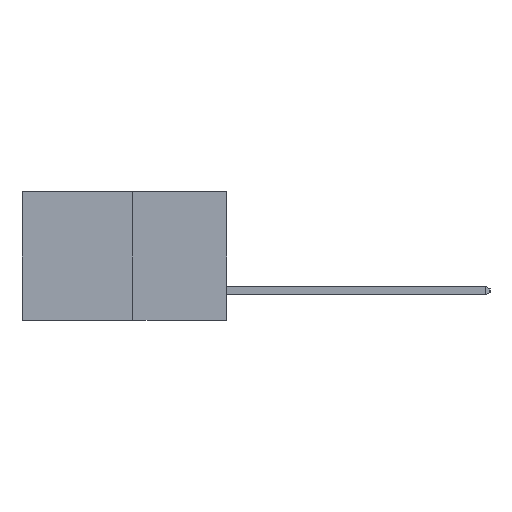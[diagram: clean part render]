
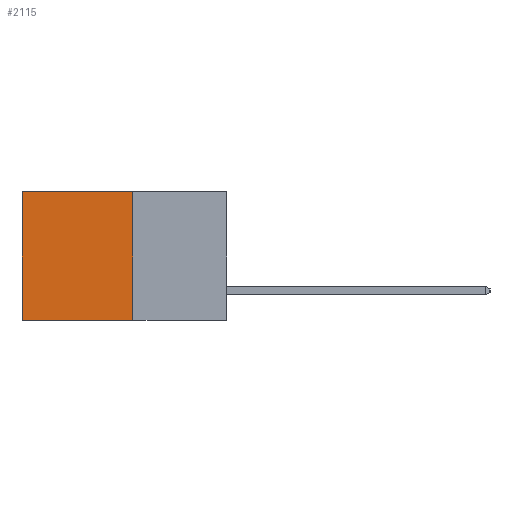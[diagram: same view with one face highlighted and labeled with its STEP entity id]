
A CAD part, left-side view. The second image highlights one B-rep face of the part: STEP entity #2115.
In plain terms, the highlighted planar face has unit normal (-1, 0, 0).
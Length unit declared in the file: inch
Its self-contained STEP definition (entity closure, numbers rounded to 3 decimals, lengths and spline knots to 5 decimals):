
#519 = ORIENTED_EDGE ( 'NONE', *, *, #10132, .F. ) ;
#786 = ORIENTED_EDGE ( 'NONE', *, *, #15309, .T. ) ;
#1230 = CARTESIAN_POINT ( 'NONE',  ( 0.277, 0.27, -0.37 ) ) ;
#1378 = ORIENTED_EDGE ( 'NONE', *, *, #7755, .F. ) ;
#1623 = EDGE_CURVE ( 'NONE', #3369, #8069, #8534, .T. ) ;
#2115 = ADVANCED_FACE ( 'NONE', ( #7200 ), #9930, .F. ) ;
#3288 = EDGE_LOOP ( 'NONE', ( #3613, #1378, #519, #786 ) ) ;
#3369 = VERTEX_POINT ( 'NONE', #16882 ) ;
#3454 = CARTESIAN_POINT ( 'NONE',  ( 0.277, 0.59, -0.37 ) ) ;
#3613 = ORIENTED_EDGE ( 'NONE', *, *, #1623, .T. ) ;
#3856 = VERTEX_POINT ( 'NONE', #1230 ) ;
#4957 = CARTESIAN_POINT ( 'NONE',  ( 0.277, 0.27, 0. ) ) ;
#7048 = DIRECTION ( 'NONE',  ( 0., 1., 0. ) ) ;
#7200 = FACE_OUTER_BOUND ( 'NONE', #3288, .T. ) ;
#7755 = EDGE_CURVE ( 'NONE', #3856, #8069, #8715, .T. ) ;
#7768 = DIRECTION ( 'NONE',  ( 0., 0., -1. ) ) ;
#8069 = VERTEX_POINT ( 'NONE', #3454 ) ;
#8168 = CARTESIAN_POINT ( 'NONE',  ( 0.277, 0.27, -0.37 ) ) ;
#8534 = LINE ( 'NONE', #10377, #15514 ) ;
#8715 = LINE ( 'NONE', #11074, #15261 ) ;
#9930 = PLANE ( 'NONE',  #12300 ) ;
#10132 = EDGE_CURVE ( 'NONE', #10457, #3856, #11898, .T. ) ;
#10377 = CARTESIAN_POINT ( 'NONE',  ( 0.277, 0.59, -0.37 ) ) ;
#10457 = VERTEX_POINT ( 'NONE', #4957 ) ;
#11048 = LINE ( 'NONE', #16785, #17589 ) ;
#11074 = CARTESIAN_POINT ( 'NONE',  ( 0.277, 0.27, -0.37 ) ) ;
#11898 = LINE ( 'NONE', #8168, #14734 ) ;
#12300 = AXIS2_PLACEMENT_3D ( 'NONE', #16145, #15002, #12659 ) ;
#12659 = DIRECTION ( 'NONE',  ( 0., 0., -1. ) ) ;
#14734 = VECTOR ( 'NONE', #15104, 39.37008 ) ;
#15002 = DIRECTION ( 'NONE',  ( 1., 0., 0. ) ) ;
#15104 = DIRECTION ( 'NONE',  ( 0., 0., -1. ) ) ;
#15261 = VECTOR ( 'NONE', #18028, 39.37008 ) ;
#15309 = EDGE_CURVE ( 'NONE', #10457, #3369, #11048, .T. ) ;
#15514 = VECTOR ( 'NONE', #7768, 39.37008 ) ;
#16145 = CARTESIAN_POINT ( 'NONE',  ( 0.277, 0.27, -0.37 ) ) ;
#16785 = CARTESIAN_POINT ( 'NONE',  ( 0.277, 0.27, 0. ) ) ;
#16882 = CARTESIAN_POINT ( 'NONE',  ( 0.277, 0.59, 0. ) ) ;
#17589 = VECTOR ( 'NONE', #7048, 39.37008 ) ;
#18028 = DIRECTION ( 'NONE',  ( 0., 1., 0. ) ) ;
